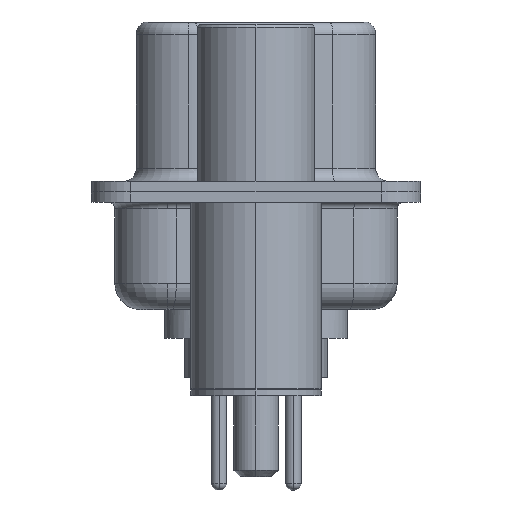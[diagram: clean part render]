
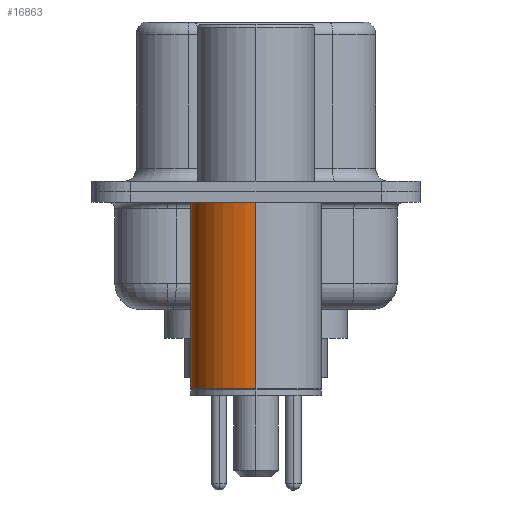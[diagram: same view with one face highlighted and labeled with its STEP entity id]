
A CAD part, left-side view. The second image highlights one B-rep face of the part: STEP entity #16863.
In plain terms, the highlighted cylindrical face has radius 2.5 mm (diameter 5 mm), a partial arc.
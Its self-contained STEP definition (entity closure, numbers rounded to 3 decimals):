
#154 = CARTESIAN_POINT ( 'NONE',  ( 2.5, 0., -0.4 ) ) ;
#591 = CARTESIAN_POINT ( 'NONE',  ( -2.5, 0., 0.581 ) ) ;
#717 = CARTESIAN_POINT ( 'NONE',  ( 0., 0., -7.525 ) ) ;
#736 = LINE ( 'NONE', #591, #15339 ) ;
#924 = VERTEX_POINT ( 'NONE', #1839 ) ;
#1839 = CARTESIAN_POINT ( 'NONE',  ( -2.5, 0., -7.525 ) ) ;
#1925 = CARTESIAN_POINT ( 'NONE',  ( 0., 0., -0.4 ) ) ;
#2742 = DIRECTION ( 'NONE',  ( 1., 0., 0. ) ) ;
#2912 = DIRECTION ( 'NONE',  ( 0., 0., 1. ) ) ;
#3055 = CYLINDRICAL_SURFACE ( 'NONE', #22085, 2.5 ) ;
#3922 = DIRECTION ( 'NONE',  ( 1., 0., 0. ) ) ;
#4248 = ORIENTED_EDGE ( 'NONE', *, *, #14879, .T. ) ;
#4603 = CARTESIAN_POINT ( 'NONE',  ( 2.5, 0., -7.525 ) ) ;
#4828 = LINE ( 'NONE', #16781, #5711 ) ;
#5711 = VECTOR ( 'NONE', #2912, 1000. ) ;
#6134 = VERTEX_POINT ( 'NONE', #154 ) ;
#8508 = DIRECTION ( 'NONE',  ( 0., 0., 1. ) ) ;
#9077 = EDGE_CURVE ( 'NONE', #924, #15862, #736, .T. ) ;
#10021 = EDGE_CURVE ( 'NONE', #6134, #15862, #18367, .T. ) ;
#10190 = DIRECTION ( 'NONE',  ( 0., 0., 1. ) ) ;
#12006 = ORIENTED_EDGE ( 'NONE', *, *, #9077, .T. ) ;
#12096 = CARTESIAN_POINT ( 'NONE',  ( 0., 0., 0.581 ) ) ;
#12274 = ORIENTED_EDGE ( 'NONE', *, *, #10021, .F. ) ;
#12617 = AXIS2_PLACEMENT_3D ( 'NONE', #1925, #15811, #3922 ) ;
#13018 = CARTESIAN_POINT ( 'NONE',  ( -2.5, 0., -0.4 ) ) ;
#13619 = FACE_OUTER_BOUND ( 'NONE', #15229, .T. ) ;
#14262 = ORIENTED_EDGE ( 'NONE', *, *, #14950, .F. ) ;
#14597 = DIRECTION ( 'NONE',  ( 0., 0., 1. ) ) ;
#14879 = EDGE_CURVE ( 'NONE', #16402, #924, #21452, .T. ) ;
#14950 = EDGE_CURVE ( 'NONE', #16402, #6134, #4828, .T. ) ;
#15229 = EDGE_LOOP ( 'NONE', ( #4248, #12006, #12274, #14262 ) ) ;
#15339 = VECTOR ( 'NONE', #8508, 1000. ) ;
#15811 = DIRECTION ( 'NONE',  ( 0., 0., 1. ) ) ;
#15862 = VERTEX_POINT ( 'NONE', #13018 ) ;
#16402 = VERTEX_POINT ( 'NONE', #4603 ) ;
#16781 = CARTESIAN_POINT ( 'NONE',  ( 2.5, 0., 0.581 ) ) ;
#16863 = ADVANCED_FACE ( 'NONE', ( #13619 ), #3055, .T. ) ;
#18367 = CIRCLE ( 'NONE', #12617, 2.5 ) ;
#21452 = CIRCLE ( 'NONE', #23316, 2.5 ) ;
#21862 = DIRECTION ( 'NONE',  ( 1., 0., 0. ) ) ;
#22085 = AXIS2_PLACEMENT_3D ( 'NONE', #12096, #10190, #21862 ) ;
#23316 = AXIS2_PLACEMENT_3D ( 'NONE', #717, #14597, #2742 ) ;
